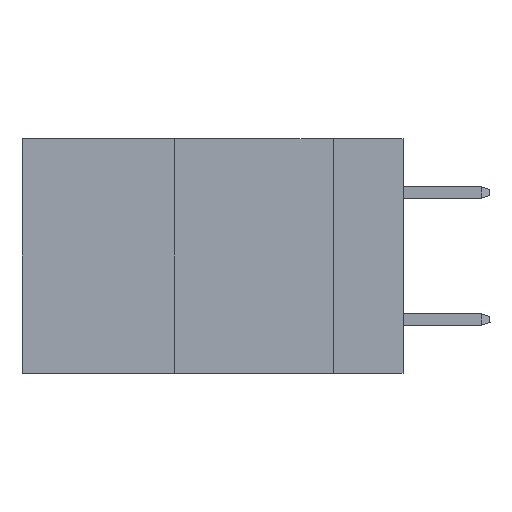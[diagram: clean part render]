
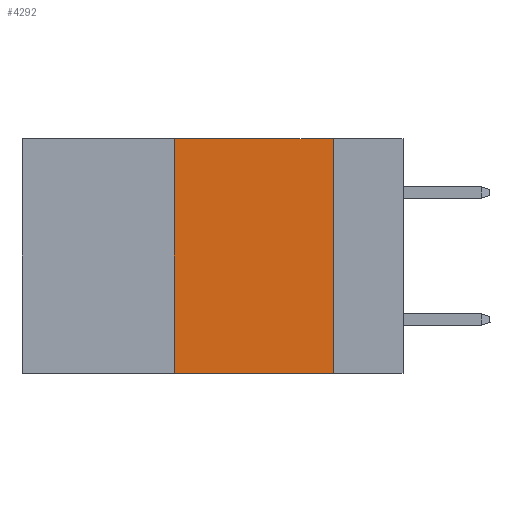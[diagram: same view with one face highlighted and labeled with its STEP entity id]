
A CAD part, left-side view. The second image highlights one B-rep face of the part: STEP entity #4292.
In plain terms, the highlighted planar face has unit normal (-1, 0, 0).
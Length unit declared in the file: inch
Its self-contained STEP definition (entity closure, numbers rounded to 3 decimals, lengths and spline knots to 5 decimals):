
#764 = CARTESIAN_POINT ( 'NONE',  ( 0., 0.36, 0. ) ) ;
#890 = EDGE_CURVE ( 'NONE', #13882, #2523, #6191, .T. ) ;
#1286 = CARTESIAN_POINT ( 'NONE',  ( 0., 0.11, -0.37 ) ) ;
#1443 = DIRECTION ( 'NONE',  ( 1., 0., 0. ) ) ;
#1522 = VECTOR ( 'NONE', #6960, 39.37008 ) ;
#2305 = ORIENTED_EDGE ( 'NONE', *, *, #890, .T. ) ;
#2523 = VERTEX_POINT ( 'NONE', #1286 ) ;
#2672 = AXIS2_PLACEMENT_3D ( 'NONE', #3459, #1443, #7849 ) ;
#3459 = CARTESIAN_POINT ( 'NONE',  ( 0., 0.6, 0. ) ) ;
#3660 = VECTOR ( 'NONE', #5272, 39.37008 ) ;
#3795 = ORIENTED_EDGE ( 'NONE', *, *, #12842, .F. ) ;
#3887 = DIRECTION ( 'NONE',  ( 0., 0., 1. ) ) ;
#4292 = ADVANCED_FACE ( 'NONE', ( #12377 ), #11306, .F. ) ;
#4415 = CARTESIAN_POINT ( 'NONE',  ( 0., 0.36, -0.37 ) ) ;
#4935 = ORIENTED_EDGE ( 'NONE', *, *, #10898, .F. ) ;
#5182 = CARTESIAN_POINT ( 'NONE',  ( 0., 0.6, -0.37 ) ) ;
#5272 = DIRECTION ( 'NONE',  ( 0., 0., -1. ) ) ;
#5316 = VECTOR ( 'NONE', #3887, 39.37008 ) ;
#6191 = LINE ( 'NONE', #5182, #8125 ) ;
#6960 = DIRECTION ( 'NONE',  ( 0., -1., 0. ) ) ;
#7409 = EDGE_CURVE ( 'NONE', #12174, #9967, #8965, .T. ) ;
#7687 = ORIENTED_EDGE ( 'NONE', *, *, #7409, .F. ) ;
#7832 = CARTESIAN_POINT ( 'NONE',  ( 0., 0.11, 0. ) ) ;
#7849 = DIRECTION ( 'NONE',  ( 0., 0., -1. ) ) ;
#8125 = VECTOR ( 'NONE', #12728, 39.37008 ) ;
#8965 = LINE ( 'NONE', #9036, #1522 ) ;
#9036 = CARTESIAN_POINT ( 'NONE',  ( 0., 0.6, 0. ) ) ;
#9349 = LINE ( 'NONE', #13728, #5316 ) ;
#9967 = VERTEX_POINT ( 'NONE', #7832 ) ;
#10594 = CARTESIAN_POINT ( 'NONE',  ( 0., 0.11, 0. ) ) ;
#10898 = EDGE_CURVE ( 'NONE', #9967, #2523, #13030, .T. ) ;
#11306 = PLANE ( 'NONE',  #2672 ) ;
#12174 = VERTEX_POINT ( 'NONE', #764 ) ;
#12224 = EDGE_LOOP ( 'NONE', ( #4935, #7687, #3795, #2305 ) ) ;
#12377 = FACE_OUTER_BOUND ( 'NONE', #12224, .T. ) ;
#12728 = DIRECTION ( 'NONE',  ( 0., -1., 0. ) ) ;
#12842 = EDGE_CURVE ( 'NONE', #13882, #12174, #9349, .T. ) ;
#13030 = LINE ( 'NONE', #10594, #3660 ) ;
#13728 = CARTESIAN_POINT ( 'NONE',  ( 0., 0.36, 0. ) ) ;
#13882 = VERTEX_POINT ( 'NONE', #4415 ) ;
